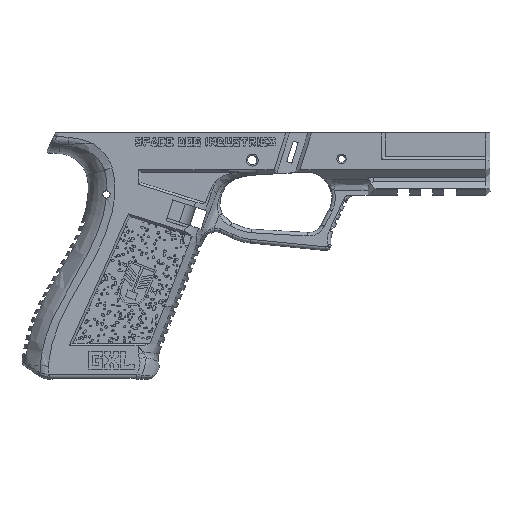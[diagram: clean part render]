
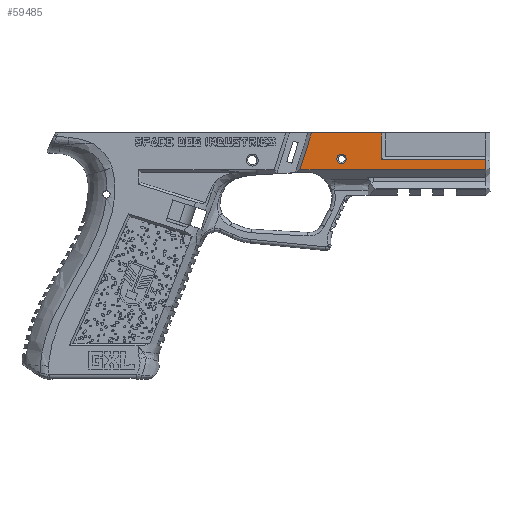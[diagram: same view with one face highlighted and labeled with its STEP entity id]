
A CAD part, top view. The second image highlights one B-rep face of the part: STEP entity #59485.
In plain terms, the highlighted planar face has unit normal (0, 0, 1).
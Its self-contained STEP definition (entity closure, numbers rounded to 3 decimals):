
#6322=FACE_BOUND('',#12833,.T.);
#8088=PLANE('',#63103);
#9233=FACE_OUTER_BOUND('',#12832,.T.);
#12832=EDGE_LOOP('',(#40658,#40659,#40660,#40661,#40662,#40663));
#12833=EDGE_LOOP('',(#40664));
#16888=LINE('',#72410,#20846);
#16894=LINE('',#72447,#20852);
#16903=LINE('',#72466,#20861);
#16904=LINE('',#72468,#20862);
#16905=LINE('',#72470,#20863);
#16906=LINE('',#72471,#20864);
#20846=VECTOR('',#64536,10.);
#20852=VECTOR('',#64546,10.);
#20861=VECTOR('',#64559,10.);
#20862=VECTOR('',#64560,10.);
#20863=VECTOR('',#64561,10.);
#20864=VECTOR('',#64562,10.);
#24802=CIRCLE('',#63104,2.025);
#24999=VERTEX_POINT('',#72407);
#25000=VERTEX_POINT('',#72409);
#25008=VERTEX_POINT('',#72445);
#25016=VERTEX_POINT('',#72465);
#25017=VERTEX_POINT('',#72467);
#25018=VERTEX_POINT('',#72469);
#25019=VERTEX_POINT('',#72472);
#31223=EDGE_CURVE('',#24999,#25000,#16888,.T.);
#31233=EDGE_CURVE('',#25008,#24999,#16894,.T.);
#31242=EDGE_CURVE('',#25016,#25008,#16903,.T.);
#31243=EDGE_CURVE('',#25016,#25017,#16904,.T.);
#31244=EDGE_CURVE('',#25018,#25017,#16905,.T.);
#31245=EDGE_CURVE('',#25000,#25018,#16906,.T.);
#31246=EDGE_CURVE('',#25019,#25019,#24802,.T.);
#40658=ORIENTED_EDGE('',*,*,#31233,.F.);
#40659=ORIENTED_EDGE('',*,*,#31242,.F.);
#40660=ORIENTED_EDGE('',*,*,#31243,.T.);
#40661=ORIENTED_EDGE('',*,*,#31244,.F.);
#40662=ORIENTED_EDGE('',*,*,#31245,.F.);
#40663=ORIENTED_EDGE('',*,*,#31223,.F.);
#40664=ORIENTED_EDGE('',*,*,#31246,.T.);
#59485=ADVANCED_FACE('',(#9233,#6322),#8088,.F.);
#63103=AXIS2_PLACEMENT_3D('',#72464,#64557,#64558);
#63104=AXIS2_PLACEMENT_3D('',#72473,#64563,#64564);
#64536=DIRECTION('',(0.301,0.954,0.));
#64546=DIRECTION('',(-1.,0.,0.));
#64557=DIRECTION('center_axis',(0.,0.,
-1.));
#64558=DIRECTION('ref_axis',(0.,1.,0.));
#64559=DIRECTION('',(0.,-1.,0.));
#64560=DIRECTION('',(-1.,0.,0.));
#64561=DIRECTION('',(0.,-1.,0.));
#64562=DIRECTION('',(1.,0.,0.));
#64563=DIRECTION('center_axis',(0.,0.,
-1.));
#64564=DIRECTION('ref_axis',(0.776,-0.63,0.));
#72407=CARTESIAN_POINT('',(77.608,-14.037,143.145));
#72409=CARTESIAN_POINT('',(82.591,1.767,143.145));
#72410=CARTESIAN_POINT('',(82.185,0.48,143.145));
#72445=CARTESIAN_POINT('',(157.385,-14.037,143.145));
#72447=CARTESIAN_POINT('',(80.448,-14.037,143.145));
#72464=CARTESIAN_POINT('Origin',(103.31,1.259,143.145));
#72465=CARTESIAN_POINT('',(157.385,-9.733,143.145));
#72466=CARTESIAN_POINT('',(157.385,-25.087,143.145));
#72467=CARTESIAN_POINT('',(112.635,-9.733,143.145));
#72468=CARTESIAN_POINT('',(105.549,-9.733,143.145));
#72469=CARTESIAN_POINT('',(112.635,1.767,143.145));
#72470=CARTESIAN_POINT('',(112.635,1.513,143.145));
#72471=CARTESIAN_POINT('',(33.317,1.767,143.145));
#72472=CARTESIAN_POINT('',(97.469,-9.398,143.145));
#72473=CARTESIAN_POINT('Origin',(95.444,-9.398,143.145));
